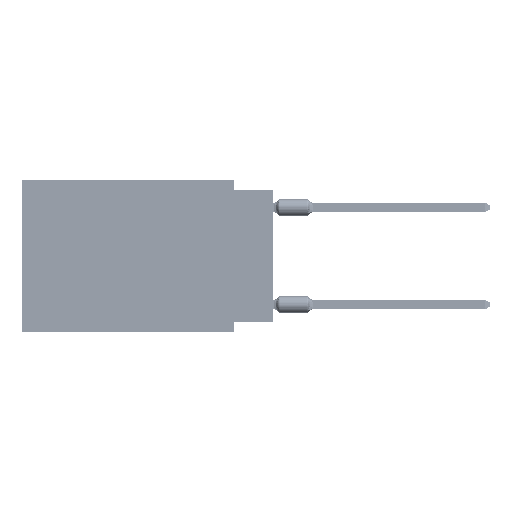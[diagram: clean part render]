
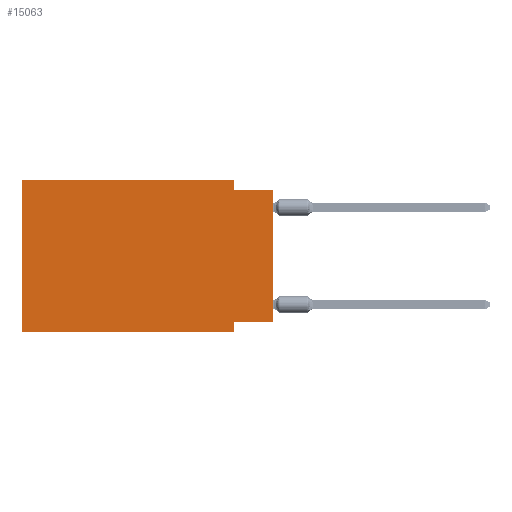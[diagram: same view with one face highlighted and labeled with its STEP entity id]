
A CAD part, left-side view. The second image highlights one B-rep face of the part: STEP entity #15063.
In plain terms, the highlighted planar face has unit normal (-1, 0, 0).
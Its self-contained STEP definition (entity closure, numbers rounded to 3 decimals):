
#1002 = VECTOR ( 'NONE', #1803, 1000. ) ;
#1803 = DIRECTION ( 'NONE',  ( 0., -1., 0. ) ) ;
#1868 = LINE ( 'NONE', #48818, #34966 ) ;
#2468 = CARTESIAN_POINT ( 'NONE',  ( 0., 2.54, -9.271 ) ) ;
#4453 = LINE ( 'NONE', #27593, #38952 ) ;
#5175 = VERTEX_POINT ( 'NONE', #56635 ) ;
#5405 = LINE ( 'NONE', #64265, #22020 ) ;
#6732 = DIRECTION ( 'NONE',  ( 0., 0., -1. ) ) ;
#7015 = CARTESIAN_POINT ( 'NONE',  ( 0., 16.383, 0. ) ) ;
#7696 = ORIENTED_EDGE ( 'NONE', *, *, #23670, .F. ) ;
#8628 = EDGE_CURVE ( 'NONE', #12679, #58465, #4453, .T. ) ;
#10721 = EDGE_CURVE ( 'NONE', #21775, #58465, #5405, .T. ) ;
#11355 = DIRECTION ( 'NONE',  ( 0., 0., 1. ) ) ;
#12679 = VERTEX_POINT ( 'NONE', #50450 ) ;
#13455 = DIRECTION ( 'NONE',  ( 0., 0., -1. ) ) ;
#13584 = CARTESIAN_POINT ( 'NONE',  ( 0., 0., -9.271 ) ) ;
#14865 = ORIENTED_EDGE ( 'NONE', *, *, #53373, .T. ) ;
#15063 = ADVANCED_FACE ( 'NONE', ( #29872 ), #35251, .F. ) ;
#16046 = EDGE_CURVE ( 'NONE', #26483, #17011, #19160, .T. ) ;
#17011 = VERTEX_POINT ( 'NONE', #42425 ) ;
#17816 = CARTESIAN_POINT ( 'NONE',  ( 0., 16.383, 0. ) ) ;
#19160 = LINE ( 'NONE', #54530, #1002 ) ;
#21304 = VERTEX_POINT ( 'NONE', #37584 ) ;
#21775 = VERTEX_POINT ( 'NONE', #2468 ) ;
#21928 = CARTESIAN_POINT ( 'NONE',  ( 0., 2.54, -0.635 ) ) ;
#22020 = VECTOR ( 'NONE', #41570, 1000. ) ;
#22170 = VERTEX_POINT ( 'NONE', #21928 ) ;
#23670 = EDGE_CURVE ( 'NONE', #21304, #21775, #60506, .T. ) ;
#26483 = VERTEX_POINT ( 'NONE', #7015 ) ;
#27593 = CARTESIAN_POINT ( 'NONE',  ( 0., 16.383, -9.906 ) ) ;
#28338 = VECTOR ( 'NONE', #58591, 1000. ) ;
#29090 = CARTESIAN_POINT ( 'NONE',  ( 0., 0., 0. ) ) ;
#29872 = FACE_OUTER_BOUND ( 'NONE', #47453, .T. ) ;
#34966 = VECTOR ( 'NONE', #13455, 1000. ) ;
#35013 = CARTESIAN_POINT ( 'NONE',  ( 0., 0., -0.635 ) ) ;
#35251 = PLANE ( 'NONE',  #45134 ) ;
#37584 = CARTESIAN_POINT ( 'NONE',  ( 0., 0., -9.271 ) ) ;
#37985 = DIRECTION ( 'NONE',  ( 0., -1., 0. ) ) ;
#38952 = VECTOR ( 'NONE', #37985, 1000. ) ;
#39013 = CARTESIAN_POINT ( 'NONE',  ( 0., 2.54, -9.906 ) ) ;
#40219 = LINE ( 'NONE', #29090, #57344 ) ;
#40240 = DIRECTION ( 'NONE',  ( 1., 0., 0. ) ) ;
#41570 = DIRECTION ( 'NONE',  ( 0., 0., -1. ) ) ;
#41960 = VECTOR ( 'NONE', #63840, 1000. ) ;
#42425 = CARTESIAN_POINT ( 'NONE',  ( 0., 2.54, 0. ) ) ;
#44311 = EDGE_CURVE ( 'NONE', #12679, #26483, #70484, .T. ) ;
#45134 = AXIS2_PLACEMENT_3D ( 'NONE', #59451, #40240, #6732 ) ;
#47453 = EDGE_LOOP ( 'NONE', ( #14865, #61841, #50968, #70735, #51188, #71451, #48249, #7696 ) ) ;
#48249 = ORIENTED_EDGE ( 'NONE', *, *, #10721, .F. ) ;
#48818 = CARTESIAN_POINT ( 'NONE',  ( 0., 2.54, 0. ) ) ;
#50450 = CARTESIAN_POINT ( 'NONE',  ( 0., 16.383, -9.906 ) ) ;
#50968 = ORIENTED_EDGE ( 'NONE', *, *, #57826, .F. ) ;
#51188 = ORIENTED_EDGE ( 'NONE', *, *, #44311, .F. ) ;
#53373 = EDGE_CURVE ( 'NONE', #21304, #5175, #40219, .T. ) ;
#54530 = CARTESIAN_POINT ( 'NONE',  ( 0., 16.383, 0. ) ) ;
#55646 = VECTOR ( 'NONE', #71645, 1000. ) ;
#56635 = CARTESIAN_POINT ( 'NONE',  ( 0., 0., -0.635 ) ) ;
#57320 = LINE ( 'NONE', #35013, #41960 ) ;
#57344 = VECTOR ( 'NONE', #11355, 1000. ) ;
#57826 = EDGE_CURVE ( 'NONE', #17011, #22170, #1868, .T. ) ;
#58465 = VERTEX_POINT ( 'NONE', #39013 ) ;
#58591 = DIRECTION ( 'NONE',  ( 0., 0., 1. ) ) ;
#59451 = CARTESIAN_POINT ( 'NONE',  ( 0., 16.383, 0. ) ) ;
#60506 = LINE ( 'NONE', #13584, #55646 ) ;
#61841 = ORIENTED_EDGE ( 'NONE', *, *, #74790, .F. ) ;
#63840 = DIRECTION ( 'NONE',  ( 0., -1., 0. ) ) ;
#64265 = CARTESIAN_POINT ( 'NONE',  ( 0., 2.54, -9.906 ) ) ;
#70484 = LINE ( 'NONE', #17816, #28338 ) ;
#70735 = ORIENTED_EDGE ( 'NONE', *, *, #16046, .F. ) ;
#71451 = ORIENTED_EDGE ( 'NONE', *, *, #8628, .T. ) ;
#71645 = DIRECTION ( 'NONE',  ( 0., 1., 0. ) ) ;
#74790 = EDGE_CURVE ( 'NONE', #22170, #5175, #57320, .T. ) ;
